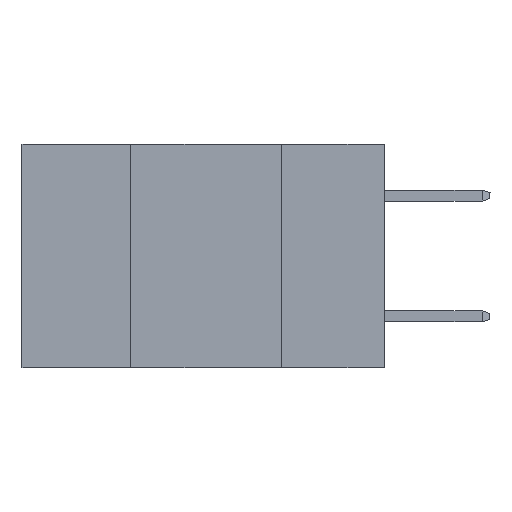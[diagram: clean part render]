
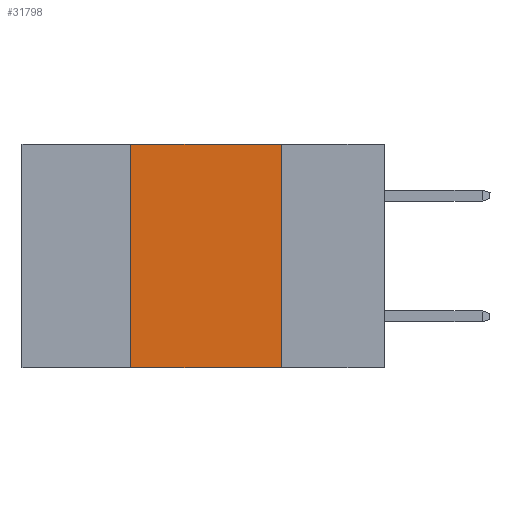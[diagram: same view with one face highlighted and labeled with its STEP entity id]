
A CAD part, left-side view. The second image highlights one B-rep face of the part: STEP entity #31798.
In plain terms, the highlighted planar face has unit normal (-1, 0, 0).
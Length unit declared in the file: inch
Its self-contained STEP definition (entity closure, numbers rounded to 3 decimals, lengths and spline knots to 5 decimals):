
#866 = CARTESIAN_POINT ( 'NONE',  ( 0., 0.6, -0.37 ) ) ;
#1594 = LINE ( 'NONE', #866, #20831 ) ;
#2080 = AXIS2_PLACEMENT_3D ( 'NONE', #29409, #31820, #17263 ) ;
#2345 = CARTESIAN_POINT ( 'NONE',  ( 0., 0.17, -0.37 ) ) ;
#3490 = DIRECTION ( 'NONE',  ( 0., -1., 0. ) ) ;
#4043 = VECTOR ( 'NONE', #13299, 39.37008 ) ;
#5263 = EDGE_LOOP ( 'NONE', ( #22768, #30218, #7119, #18001 ) ) ;
#6498 = VERTEX_POINT ( 'NONE', #10491 ) ;
#7119 = ORIENTED_EDGE ( 'NONE', *, *, #21800, .F. ) ;
#7535 = CARTESIAN_POINT ( 'NONE',  ( 0., 0.42, -0.37 ) ) ;
#8402 = DIRECTION ( 'NONE',  ( 0., 0., 1. ) ) ;
#10491 = CARTESIAN_POINT ( 'NONE',  ( 0., 0.17, 0. ) ) ;
#10795 = CARTESIAN_POINT ( 'NONE',  ( 0., 0.6, 0. ) ) ;
#10915 = LINE ( 'NONE', #10795, #4043 ) ;
#11482 = CARTESIAN_POINT ( 'NONE',  ( 0., 0.42, 0. ) ) ;
#12392 = PLANE ( 'NONE',  #2080 ) ;
#13299 = DIRECTION ( 'NONE',  ( 0., -1., 0. ) ) ;
#13809 = VERTEX_POINT ( 'NONE', #7535 ) ;
#15316 = EDGE_CURVE ( 'NONE', #13809, #20362, #1594, .T. ) ;
#16040 = CARTESIAN_POINT ( 'NONE',  ( 0., 0.42, 0. ) ) ;
#17263 = DIRECTION ( 'NONE',  ( 0., 0., -1. ) ) ;
#17728 = EDGE_CURVE ( 'NONE', #22834, #6498, #10915, .T. ) ;
#18001 = ORIENTED_EDGE ( 'NONE', *, *, #15316, .T. ) ;
#18882 = CARTESIAN_POINT ( 'NONE',  ( 0., 0.17, 0. ) ) ;
#19456 = VECTOR ( 'NONE', #8402, 39.37008 ) ;
#20362 = VERTEX_POINT ( 'NONE', #2345 ) ;
#20831 = VECTOR ( 'NONE', #3490, 39.37008 ) ;
#21790 = VECTOR ( 'NONE', #31050, 39.37008 ) ;
#21800 = EDGE_CURVE ( 'NONE', #13809, #22834, #23629, .T. ) ;
#22768 = ORIENTED_EDGE ( 'NONE', *, *, #23390, .F. ) ;
#22834 = VERTEX_POINT ( 'NONE', #11482 ) ;
#23390 = EDGE_CURVE ( 'NONE', #6498, #20362, #28263, .T. ) ;
#23629 = LINE ( 'NONE', #16040, #19456 ) ;
#25834 = FACE_OUTER_BOUND ( 'NONE', #5263, .T. ) ;
#28263 = LINE ( 'NONE', #18882, #21790 ) ;
#29409 = CARTESIAN_POINT ( 'NONE',  ( 0., 0.6, 0. ) ) ;
#30218 = ORIENTED_EDGE ( 'NONE', *, *, #17728, .F. ) ;
#31050 = DIRECTION ( 'NONE',  ( 0., 0., -1. ) ) ;
#31798 = ADVANCED_FACE ( 'NONE', ( #25834 ), #12392, .F. ) ;
#31820 = DIRECTION ( 'NONE',  ( 1., 0., 0. ) ) ;
